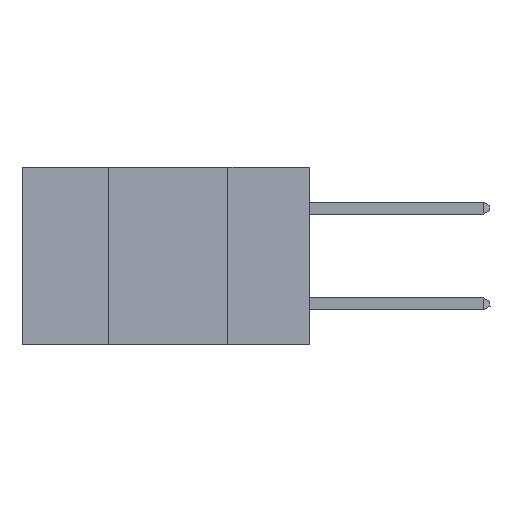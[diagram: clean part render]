
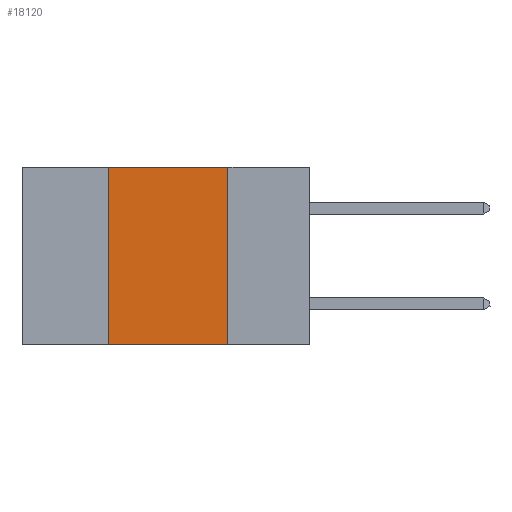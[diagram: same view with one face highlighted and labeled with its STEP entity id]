
A CAD part, left-side view. The second image highlights one B-rep face of the part: STEP entity #18120.
In plain terms, the highlighted planar face has unit normal (-1, 0, 0).
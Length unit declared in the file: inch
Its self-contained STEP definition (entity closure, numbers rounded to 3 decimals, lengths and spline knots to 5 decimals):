
#383 = VECTOR ( 'NONE', #1690, 39.37008 ) ;
#1690 = DIRECTION ( 'NONE',  ( 0., -1., 0. ) ) ;
#2478 = LINE ( 'NONE', #20735, #24031 ) ;
#2497 = VECTOR ( 'NONE', #5477, 39.37008 ) ;
#3482 = DIRECTION ( 'NONE',  ( 0., 0., -1. ) ) ;
#3712 = VECTOR ( 'NONE', #9761, 39.37008 ) ;
#5209 = DIRECTION ( 'NONE',  ( 0., 0., -1. ) ) ;
#5477 = DIRECTION ( 'NONE',  ( 0., -1., 0. ) ) ;
#6527 = LINE ( 'NONE', #7667, #3712 ) ;
#7667 = CARTESIAN_POINT ( 'NONE',  ( 0., 0.42, 0. ) ) ;
#7987 = CARTESIAN_POINT ( 'NONE',  ( 0., 0.42, 0. ) ) ;
#8868 = EDGE_CURVE ( 'NONE', #24030, #9868, #2478, .T. ) ;
#9687 = CARTESIAN_POINT ( 'NONE',  ( 0., 0.6, -0.37 ) ) ;
#9761 = DIRECTION ( 'NONE',  ( 0., 0., 1. ) ) ;
#9868 = VERTEX_POINT ( 'NONE', #25478 ) ;
#10561 = VERTEX_POINT ( 'NONE', #7987 ) ;
#11640 = DIRECTION ( 'NONE',  ( 1., 0., 0. ) ) ;
#13011 = EDGE_CURVE ( 'NONE', #14640, #9868, #16046, .T. ) ;
#13467 = CARTESIAN_POINT ( 'NONE',  ( 0., 0.17, 0. ) ) ;
#13569 = EDGE_LOOP ( 'NONE', ( #21266, #21886, #20476, #20072 ) ) ;
#14264 = CARTESIAN_POINT ( 'NONE',  ( 0., 0.42, -0.37 ) ) ;
#14640 = VERTEX_POINT ( 'NONE', #14264 ) ;
#16046 = LINE ( 'NONE', #9687, #383 ) ;
#16627 = EDGE_CURVE ( 'NONE', #14640, #10561, #6527, .T. ) ;
#17422 = CARTESIAN_POINT ( 'NONE',  ( 0., 0.6, 0. ) ) ;
#17714 = FACE_OUTER_BOUND ( 'NONE', #13569, .T. ) ;
#18120 = ADVANCED_FACE ( 'NONE', ( #17714 ), #19483, .F. ) ;
#18462 = LINE ( 'NONE', #17422, #2497 ) ;
#19483 = PLANE ( 'NONE',  #21024 ) ;
#20072 = ORIENTED_EDGE ( 'NONE', *, *, #13011, .T. ) ;
#20476 = ORIENTED_EDGE ( 'NONE', *, *, #16627, .F. ) ;
#20735 = CARTESIAN_POINT ( 'NONE',  ( 0., 0.17, 0. ) ) ;
#21024 = AXIS2_PLACEMENT_3D ( 'NONE', #25733, #11640, #3482 ) ;
#21266 = ORIENTED_EDGE ( 'NONE', *, *, #8868, .F. ) ;
#21886 = ORIENTED_EDGE ( 'NONE', *, *, #25474, .F. ) ;
#24030 = VERTEX_POINT ( 'NONE', #13467 ) ;
#24031 = VECTOR ( 'NONE', #5209, 39.37008 ) ;
#25474 = EDGE_CURVE ( 'NONE', #10561, #24030, #18462, .T. ) ;
#25478 = CARTESIAN_POINT ( 'NONE',  ( 0., 0.17, -0.37 ) ) ;
#25733 = CARTESIAN_POINT ( 'NONE',  ( 0., 0.6, 0. ) ) ;
